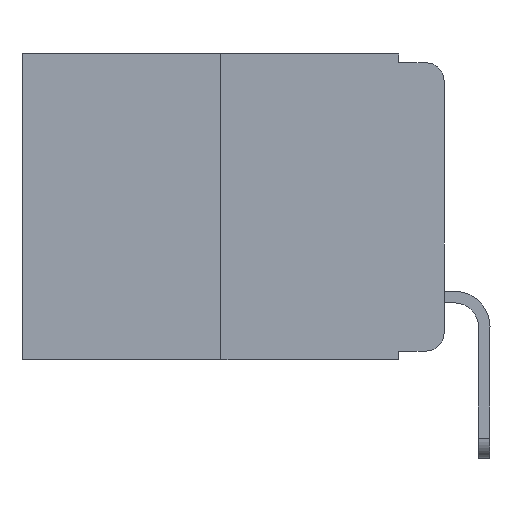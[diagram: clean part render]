
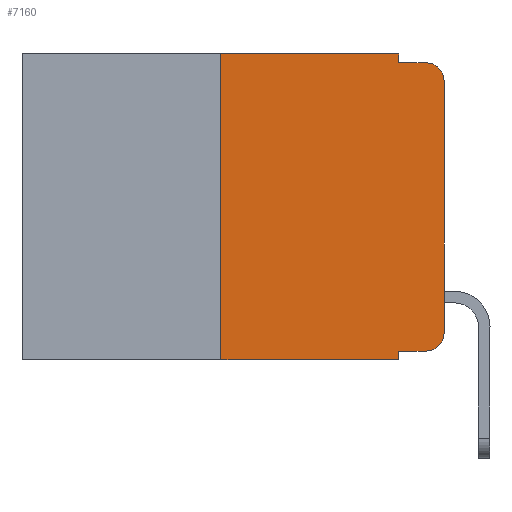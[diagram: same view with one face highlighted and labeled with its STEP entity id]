
A CAD part, left-side view. The second image highlights one B-rep face of the part: STEP entity #7160.
In plain terms, the highlighted planar face has unit normal (-1, 0, 0).
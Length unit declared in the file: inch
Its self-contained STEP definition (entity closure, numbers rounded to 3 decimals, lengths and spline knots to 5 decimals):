
#297 = ORIENTED_EDGE ( 'NONE', *, *, #4731, .T. ) ;
#428 = DIRECTION ( 'NONE',  ( -1., 0., 0. ) ) ;
#511 = CARTESIAN_POINT ( 'NONE',  ( 0., 0.25, -0.343 ) ) ;
#524 = ORIENTED_EDGE ( 'NONE', *, *, #4869, .T. ) ;
#630 = AXIS2_PLACEMENT_3D ( 'NONE', #8095, #428, #6638 ) ;
#649 = VERTEX_POINT ( 'NONE', #12357 ) ;
#703 = VERTEX_POINT ( 'NONE', #5082 ) ;
#763 = ORIENTED_EDGE ( 'NONE', *, *, #4798, .F. ) ;
#786 = PLANE ( 'NONE',  #10447 ) ;
#1126 = AXIS2_PLACEMENT_3D ( 'NONE', #3684, #3749, #4886 ) ;
#1270 = ORIENTED_EDGE ( 'NONE', *, *, #4754, .F. ) ;
#1451 = LINE ( 'NONE', #7933, #11361 ) ;
#1454 = ORIENTED_EDGE ( 'NONE', *, *, #4691, .T. ) ;
#1525 = ORIENTED_EDGE ( 'NONE', *, *, #5861, .F. ) ;
#1643 = DIRECTION ( 'NONE',  ( 0., 0., 1. ) ) ;
#1799 = LINE ( 'NONE', #11268, #9715 ) ;
#1814 = ORIENTED_EDGE ( 'NONE', *, *, #4734, .F. ) ;
#2257 = CIRCLE ( 'NONE', #630, 0.02 ) ;
#2446 = CIRCLE ( 'NONE', #1126, 0.02 ) ;
#2608 = LINE ( 'NONE', #6953, #10097 ) ;
#2658 = ORIENTED_EDGE ( 'NONE', *, *, #4846, .T. ) ;
#2839 = CARTESIAN_POINT ( 'NONE',  ( 0., 0.473, 0. ) ) ;
#2850 = DIRECTION ( 'NONE',  ( 0., -1., 0. ) ) ;
#3030 = VECTOR ( 'NONE', #11969, 39.37008 ) ;
#3107 = EDGE_LOOP ( 'NONE', ( #2658, #524, #763, #1270, #1525, #1814, #6131, #5172, #297, #1454 ) ) ;
#3549 = CARTESIAN_POINT ( 'NONE',  ( 0., 0., -0.313 ) ) ;
#3573 = CARTESIAN_POINT ( 'NONE',  ( 0., 0.051, -0.343 ) ) ;
#3684 = CARTESIAN_POINT ( 'NONE',  ( 0., 0.02, -0.313 ) ) ;
#3749 = DIRECTION ( 'NONE',  ( -1., 0., 0. ) ) ;
#3775 = DIRECTION ( 'NONE',  ( 0., 0., -1. ) ) ;
#3918 = VECTOR ( 'NONE', #3775, 39.37008 ) ;
#4069 = CARTESIAN_POINT ( 'NONE',  ( 0., 0.051, -0.333 ) ) ;
#4540 = VERTEX_POINT ( 'NONE', #6044 ) ;
#4627 = VERTEX_POINT ( 'NONE', #4979 ) ;
#4691 = EDGE_CURVE ( 'NONE', #4627, #7232, #2446, .T. ) ;
#4731 = EDGE_CURVE ( 'NONE', #6030, #4627, #11838, .T. ) ;
#4734 = EDGE_CURVE ( 'NONE', #8265, #8122, #4917, .T. ) ;
#4748 = EDGE_CURVE ( 'NONE', #6030, #11497, #1451, .T. ) ;
#4754 = EDGE_CURVE ( 'NONE', #649, #703, #9465, .T. ) ;
#4761 = CARTESIAN_POINT ( 'NONE',  ( 0., 0.473, -0.343 ) ) ;
#4798 = EDGE_CURVE ( 'NONE', #703, #5019, #10638, .T. ) ;
#4846 = EDGE_CURVE ( 'NONE', #7232, #4540, #2608, .T. ) ;
#4869 = EDGE_CURVE ( 'NONE', #4540, #5019, #2257, .T. ) ;
#4886 = DIRECTION ( 'NONE',  ( 0., 0., -1. ) ) ;
#4917 = LINE ( 'NONE', #11296, #6964 ) ;
#4979 = CARTESIAN_POINT ( 'NONE',  ( 0., 0.02, -0.333 ) ) ;
#5019 = VERTEX_POINT ( 'NONE', #7073 ) ;
#5030 = FACE_OUTER_BOUND ( 'NONE', #3107, .T. ) ;
#5082 = CARTESIAN_POINT ( 'NONE',  ( 0., 0.051, -0.01 ) ) ;
#5172 = ORIENTED_EDGE ( 'NONE', *, *, #4748, .F. ) ;
#5861 = EDGE_CURVE ( 'NONE', #8122, #649, #1799, .T. ) ;
#6030 = VERTEX_POINT ( 'NONE', #7207 ) ;
#6044 = CARTESIAN_POINT ( 'NONE',  ( 0., 0., -0.03 ) ) ;
#6129 = LINE ( 'NONE', #4761, #3030 ) ;
#6131 = ORIENTED_EDGE ( 'NONE', *, *, #10514, .T. ) ;
#6638 = DIRECTION ( 'NONE',  ( 0., 0., -1. ) ) ;
#6953 = CARTESIAN_POINT ( 'NONE',  ( 0., 0., 0. ) ) ;
#6964 = VECTOR ( 'NONE', #1643, 39.37008 ) ;
#6991 = DIRECTION ( 'NONE',  ( 0., 0., 1. ) ) ;
#7073 = CARTESIAN_POINT ( 'NONE',  ( 0., 0.02, -0.01 ) ) ;
#7160 = ADVANCED_FACE ( 'NONE', ( #5030 ), #786, .F. ) ;
#7207 = CARTESIAN_POINT ( 'NONE',  ( 0., 0.051, -0.333 ) ) ;
#7232 = VERTEX_POINT ( 'NONE', #3549 ) ;
#7376 = DIRECTION ( 'NONE',  ( 0., 0., -1. ) ) ;
#7561 = DIRECTION ( 'NONE',  ( 0., 0., -1. ) ) ;
#7676 = CARTESIAN_POINT ( 'NONE',  ( 0., 0.25, 0. ) ) ;
#7933 = CARTESIAN_POINT ( 'NONE',  ( 0., 0.051, 0. ) ) ;
#7948 = DIRECTION ( 'NONE',  ( 0., -1., 0. ) ) ;
#8009 = CARTESIAN_POINT ( 'NONE',  ( 0., 0.051, -0.01 ) ) ;
#8095 = CARTESIAN_POINT ( 'NONE',  ( 0., 0.02, -0.03 ) ) ;
#8122 = VERTEX_POINT ( 'NONE', #7676 ) ;
#8181 = DIRECTION ( 'NONE',  ( 0., -1., 0. ) ) ;
#8265 = VERTEX_POINT ( 'NONE', #511 ) ;
#8325 = DIRECTION ( 'NONE',  ( 1., 0., 0. ) ) ;
#8354 = VECTOR ( 'NONE', #7948, 39.37008 ) ;
#9465 = LINE ( 'NONE', #10395, #3918 ) ;
#9715 = VECTOR ( 'NONE', #8181, 39.37008 ) ;
#10097 = VECTOR ( 'NONE', #6991, 39.37008 ) ;
#10395 = CARTESIAN_POINT ( 'NONE',  ( 0., 0.051, 0. ) ) ;
#10447 = AXIS2_PLACEMENT_3D ( 'NONE', #2839, #8325, #7376 ) ;
#10514 = EDGE_CURVE ( 'NONE', #8265, #11497, #6129, .T. ) ;
#10638 = LINE ( 'NONE', #8009, #8354 ) ;
#11268 = CARTESIAN_POINT ( 'NONE',  ( 0., 0.473, 0. ) ) ;
#11296 = CARTESIAN_POINT ( 'NONE',  ( 0., 0.25, 0. ) ) ;
#11361 = VECTOR ( 'NONE', #7561, 39.37008 ) ;
#11497 = VERTEX_POINT ( 'NONE', #3573 ) ;
#11600 = VECTOR ( 'NONE', #2850, 39.37008 ) ;
#11838 = LINE ( 'NONE', #4069, #11600 ) ;
#11969 = DIRECTION ( 'NONE',  ( 0., -1., 0. ) ) ;
#12357 = CARTESIAN_POINT ( 'NONE',  ( 0., 0.051, 0. ) ) ;
